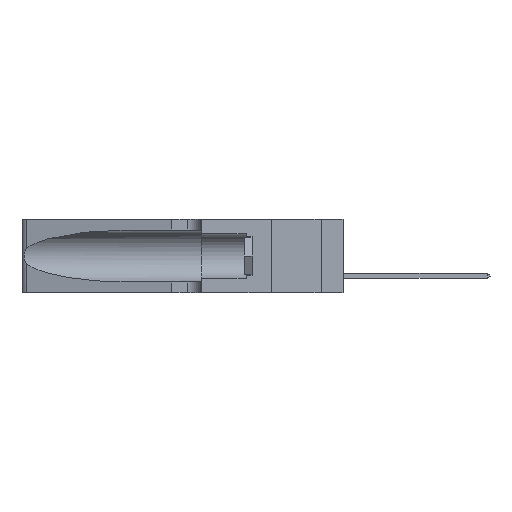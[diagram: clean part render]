
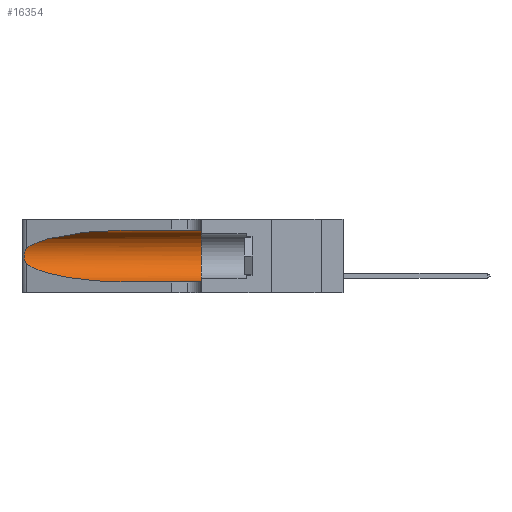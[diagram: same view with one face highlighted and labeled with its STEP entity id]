
A CAD part, left-side view. The second image highlights one B-rep face of the part: STEP entity #16354.
In plain terms, the highlighted cylindrical face has radius 3.308 mm (diameter 6.617 mm), a partial arc.
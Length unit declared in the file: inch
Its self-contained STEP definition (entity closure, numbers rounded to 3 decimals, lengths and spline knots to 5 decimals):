
#1286 = CARTESIAN_POINT ( 'NONE',  ( 0.1305, 0.72297, 0.05475 ) ) ;
#1331 = EDGE_CURVE ( 'NONE', #30386, #25594, #21577, .T. ) ;
#1881 = CARTESIAN_POINT ( 'NONE',  ( 0.26075, 1.23896, 0.19203 ) ) ;
#2507 = LINE ( 'NONE', #22374, #20460 ) ;
#2614 = CARTESIAN_POINT ( 'NONE',  ( 0.25487, 1.22718, 0.14631 ) ) ;
#3251 = CARTESIAN_POINT ( 'NONE',  ( 0.2373, 1.15595, 0.28018 ) ) ;
#3397 = DIRECTION ( 'NONE',  ( 0., -1., 0. ) ) ;
#4569 = CARTESIAN_POINT ( 'NONE',  ( 0.25639, 1.23184, 0.21858 ) ) ;
#4667 = CARTESIAN_POINT ( 'NONE',  ( 0.25555, 1.22994, 0.2215 ) ) ;
#4818 = DIRECTION ( 'NONE',  ( 0., 0., 1. ) ) ;
#5086 = CARTESIAN_POINT ( 'NONE',  ( 0.1305, 0.72297, 0.05475 ) ) ;
#5303 = CARTESIAN_POINT ( 'NONE',  ( 0.2373, 1.15595, 0.08982 ) ) ;
#6715 = CARTESIAN_POINT ( 'NONE',  ( 0.25854, 1.2359, 0.20912 ) ) ;
#6825 = CARTESIAN_POINT ( 'NONE',  ( 0.26017, 1.23833, 0.17102 ) ) ;
#7045 = CARTESIAN_POINT ( 'NONE',  ( 0.25787, 1.23484, 0.2124 ) ) ;
#8734 = LINE ( 'NONE', #26013, #22025 ) ;
#9322 = AXIS2_PLACEMENT_3D ( 'NONE', #27569, #24984, #16081 ) ;
#9483 = CARTESIAN_POINT ( 'NONE',  ( 0.25639, 1.23186, 0.15144 ) ) ;
#9806 = CARTESIAN_POINT ( 'NONE',  ( 0.1305, 0.35, 0.05475 ) ) ;
#10469 = CARTESIAN_POINT ( 'NONE',  ( 0.25487, 1.22718, 0.22369 ) ) ;
#10470 = CARTESIAN_POINT ( 'NONE',  ( 0.1305, 0.72297, 0.31525 ) ) ;
#10492 = VERTEX_POINT ( 'NONE', #16677 ) ;
#11767 = ORIENTED_EDGE ( 'NONE', *, *, #28844, .T. ) ;
#11889 = CARTESIAN_POINT ( 'NONE',  ( 0.25487, 1.22718, 0.14631 ) ) ;
#12933 = CARTESIAN_POINT ( 'NONE',  ( 0.18966, 0.96281, 0.31525 ) ) ;
#13001 = EDGE_CURVE ( 'NONE', #31156, #10492, #2507, .T. ) ;
#13311 = VERTEX_POINT ( 'NONE', #10469 ) ;
#15471 = CARTESIAN_POINT ( 'NONE',  ( 0.25487, 1.22718, 0.22369 ) ) ;
#16081 = DIRECTION ( 'NONE',  ( 0., 0., -1. ) ) ;
#16354 = ADVANCED_FACE ( 'NONE', ( #30938 ), #20728, .F. ) ;
#16586 = CARTESIAN_POINT ( 'NONE',  ( 0.25789, 1.23486, 0.15765 ) ) ;
#16677 = CARTESIAN_POINT ( 'NONE',  ( 0.1305, 0.35, 0.31525 ) ) ;
#18093 = ORIENTED_EDGE ( 'NONE', *, *, #13001, .F. ) ;
#18915 = EDGE_CURVE ( 'NONE', #31156, #13311, #31419, .T. ) ;
#19146 = CARTESIAN_POINT ( 'NONE',  ( 0.25487, 1.22718, 0.22369 ) ) ;
#20331 = EDGE_LOOP ( 'NONE', ( #21063, #11767, #29975, #21752, #25782, #18093 ) ) ;
#20460 = VECTOR ( 'NONE', #3397, 39.37008 ) ;
#20728 = CYLINDRICAL_SURFACE ( 'NONE', #9322, 0.13025 ) ;
#21063 = ORIENTED_EDGE ( 'NONE', *, *, #18915, .T. ) ;
#21266 = AXIS2_PLACEMENT_3D ( 'NONE', #31146, #21558, #4818 ) ;
#21414 = CARTESIAN_POINT ( 'NONE',  ( 0.26075, 1.23896, 0.178 ) ) ;
#21558 = DIRECTION ( 'NONE',  ( 0., 1., 0. ) ) ;
#21577 =( BOUNDED_CURVE ( )  B_SPLINE_CURVE ( 3, ( #2614, #5303, #29385, #5086 ),
 .UNSPECIFIED., .F., .T. ) 
 B_SPLINE_CURVE_WITH_KNOTS ( ( 4, 4 ),
 ( 3.44316, 4.71239 ),
 .UNSPECIFIED. ) 
 CURVE ( )  GEOMETRIC_REPRESENTATION_ITEM ( )  RATIONAL_B_SPLINE_CURVE ( ( 1., 0.87, 0.87, 1. ) ) 
 REPRESENTATION_ITEM ( '' )  );
#21752 = ORIENTED_EDGE ( 'NONE', *, *, #22956, .T. ) ;
#22025 = VECTOR ( 'NONE', #26126, 39.37008 ) ;
#22374 = CARTESIAN_POINT ( 'NONE',  ( 0.1305, 1.61858, 0.31525 ) ) ;
#22441 = EDGE_CURVE ( 'NONE', #10492, #24920, #26245, .T. ) ;
#22956 = EDGE_CURVE ( 'NONE', #25594, #24920, #8734, .T. ) ;
#24059 = CARTESIAN_POINT ( 'NONE',  ( 0.26018, 1.23835, 0.19895 ) ) ;
#24888 = B_SPLINE_CURVE_WITH_KNOTS ( 'NONE', 3,
 ( #19146, #4667, #4569, #7045, #6715, #24059, #1881, #21414, #6825, #26262, #16586, #9483, #26459, #28862 ),
 .UNSPECIFIED., .F., .F.,
 ( 4, 2, 2, 2, 2, 2, 4 ),
 ( 0., 0.00027, 0.00053, 0.00107, 0.0016, 0.00187, 0.00214 ),
 .UNSPECIFIED. ) ;
#24920 = VERTEX_POINT ( 'NONE', #9806 ) ;
#24984 = DIRECTION ( 'NONE',  ( 0., -1., 0. ) ) ;
#25594 = VERTEX_POINT ( 'NONE', #1286 ) ;
#25782 = ORIENTED_EDGE ( 'NONE', *, *, #22441, .F. ) ;
#26013 = CARTESIAN_POINT ( 'NONE',  ( 0.1305, 1.61858, 0.05475 ) ) ;
#26126 = DIRECTION ( 'NONE',  ( 0., -1., 0. ) ) ;
#26245 = CIRCLE ( 'NONE', #21266, 0.13025 ) ;
#26262 = CARTESIAN_POINT ( 'NONE',  ( 0.25856, 1.23593, 0.16098 ) ) ;
#26459 = CARTESIAN_POINT ( 'NONE',  ( 0.25555, 1.22993, 0.14849 ) ) ;
#27491 = CARTESIAN_POINT ( 'NONE',  ( 0.1305, 0.72297, 0.31525 ) ) ;
#27569 = CARTESIAN_POINT ( 'NONE',  ( 0.1305, 1.61858, 0.185 ) ) ;
#28844 = EDGE_CURVE ( 'NONE', #13311, #30386, #24888, .T. ) ;
#28862 = CARTESIAN_POINT ( 'NONE',  ( 0.25487, 1.22718, 0.14631 ) ) ;
#29385 = CARTESIAN_POINT ( 'NONE',  ( 0.18966, 0.96281, 0.05475 ) ) ;
#29975 = ORIENTED_EDGE ( 'NONE', *, *, #1331, .T. ) ;
#30386 = VERTEX_POINT ( 'NONE', #11889 ) ;
#30938 = FACE_OUTER_BOUND ( 'NONE', #20331, .T. ) ;
#31146 = CARTESIAN_POINT ( 'NONE',  ( 0.1305, 0.35, 0.185 ) ) ;
#31156 = VERTEX_POINT ( 'NONE', #10470 ) ;
#31419 =( BOUNDED_CURVE ( )  B_SPLINE_CURVE ( 3, ( #27491, #12933, #3251, #15471 ),
 .UNSPECIFIED., .F., .T. ) 
 B_SPLINE_CURVE_WITH_KNOTS ( ( 4, 4 ),
 ( 1.5708, 2.84003 ),
 .UNSPECIFIED. ) 
 CURVE ( )  GEOMETRIC_REPRESENTATION_ITEM ( )  RATIONAL_B_SPLINE_CURVE ( ( 1., 0.87, 0.87, 1. ) ) 
 REPRESENTATION_ITEM ( '' )  );
